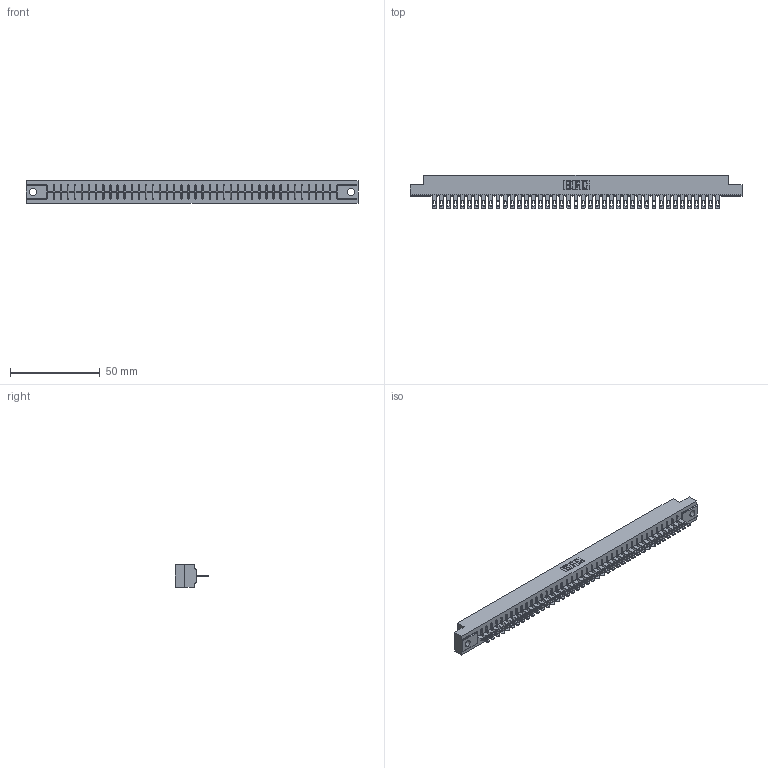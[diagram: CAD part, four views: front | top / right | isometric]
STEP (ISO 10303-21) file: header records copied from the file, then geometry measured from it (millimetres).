
FILE_DESCRIPTION (( 'STEP AP203' ), '1' );
FILE_NAME ('316-041-400-104.STEP', '2020-09-23T06:58:09', ( '' ), ( '' ), 'SwSTEP 2.0', 'SolidWorks 2020', '' );
FILE_SCHEMA (( 'CONFIG_CONTROL_DESIGN' ));
Length unit declared in the file: inch
Products named in the file (3): 306 Part_.156 Dia; 306-290-001_100; 316-041-400-104
Assembly tree (42 placements, depth 2):
  316-041-400-104
    306 Part_.156 Dia
    306-290-001_100  x41
Bounding box: 185.47 x 18.87 x 12.7 mm (x, y, z)
Volume: 20535.8 mm3; surface area: 21593.4 mm2
Topology: 42 solids, 42 shells, 3246 faces, 9167 edges, 5890 vertices
Faces by surface type: plane 2132, cylinder 950, sphere 164
Entity records: 38946 total; most frequent: CARTESIAN_POINT 6544, ORIENTED_EDGE 6486, DIRECTION 6445, EDGE_CURVE 3243, VECTOR 2543, LINE 2543, VERTEX_POINT 2050, AXIS2_PLACEMENT_3D 1951
